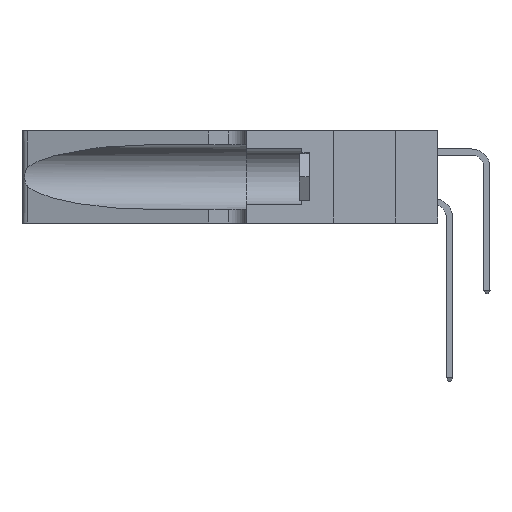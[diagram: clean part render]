
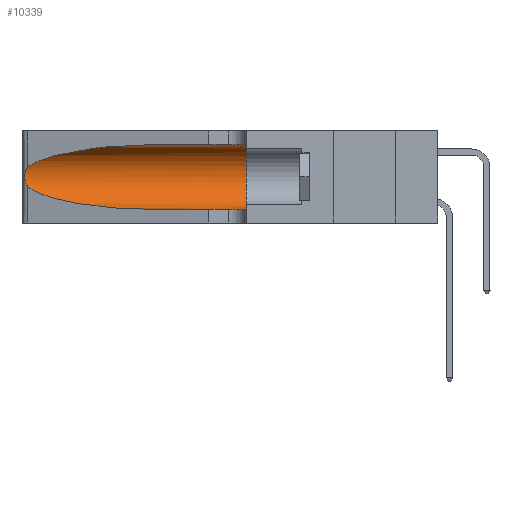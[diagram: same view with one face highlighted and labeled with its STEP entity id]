
A CAD part, left-side view. The second image highlights one B-rep face of the part: STEP entity #10339.
In plain terms, the highlighted cylindrical face has radius 3.308 mm (diameter 6.617 mm), a partial arc.
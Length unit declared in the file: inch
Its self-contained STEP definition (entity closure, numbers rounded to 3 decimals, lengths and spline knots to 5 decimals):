
#837 =( BOUNDED_CURVE ( )  B_SPLINE_CURVE ( 3, ( #22270, #9101, #14815, #3333 ),
 .UNSPECIFIED., .F., .T. ) 
 B_SPLINE_CURVE_WITH_KNOTS ( ( 4, 4 ),
 ( 1.5708, 2.84003 ),
 .UNSPECIFIED. ) 
 CURVE ( )  GEOMETRIC_REPRESENTATION_ITEM ( )  RATIONAL_B_SPLINE_CURVE ( ( 1., 0.87, 0.87, 1. ) ) 
 REPRESENTATION_ITEM ( '' )  );
#998 = EDGE_CURVE ( 'NONE', #23473, #14423, #1477, .T. ) ;
#1050 = ORIENTED_EDGE ( 'NONE', *, *, #11683, .T. ) ;
#1198 = EDGE_CURVE ( 'NONE', #12039, #12896, #8550, .T. ) ;
#1477 = B_SPLINE_CURVE_WITH_KNOTS ( 'NONE', 3,
 ( #12448, #19894, #19383, #19807, #13295, #18760, #21488, #17573, #22942, #7159, #22760, #13082, #13023, #12471 ),
 .UNSPECIFIED., .F., .F.,
 ( 4, 2, 2, 2, 2, 2, 4 ),
 ( 0., 0.00027, 0.00053, 0.00107, 0.0016, 0.00187, 0.00214 ),
 .UNSPECIFIED. ) ;
#3090 = EDGE_CURVE ( 'NONE', #20179, #12896, #11149, .T. ) ;
#3333 = CARTESIAN_POINT ( 'NONE',  ( 0.25487, 1.22718, 0.22369 ) ) ;
#4627 = CARTESIAN_POINT ( 'NONE',  ( 0.1305, 0.72297, 0.05475 ) ) ;
#5483 = CARTESIAN_POINT ( 'NONE',  ( 0.25487, 1.22718, 0.14631 ) ) ;
#5900 = ORIENTED_EDGE ( 'NONE', *, *, #1198, .T. ) ;
#6543 = CARTESIAN_POINT ( 'NONE',  ( 0.1305, 1.61858, 0.185 ) ) ;
#7159 = CARTESIAN_POINT ( 'NONE',  ( 0.25856, 1.23593, 0.16098 ) ) ;
#7175 = ORIENTED_EDGE ( 'NONE', *, *, #23449, .F. ) ;
#7817 = CARTESIAN_POINT ( 'NONE',  ( 0.1305, 1.61858, 0.05475 ) ) ;
#8189 = AXIS2_PLACEMENT_3D ( 'NONE', #20800, #9505, #22675 ) ;
#8471 = DIRECTION ( 'NONE',  ( 0., -1., 0. ) ) ;
#8550 = LINE ( 'NONE', #7817, #22967 ) ;
#9101 = CARTESIAN_POINT ( 'NONE',  ( 0.18966, 0.96281, 0.31525 ) ) ;
#9147 = EDGE_LOOP ( 'NONE', ( #11812, #12582, #1050, #5900, #21567, #7175 ) ) ;
#9505 = DIRECTION ( 'NONE',  ( 0., 1., 0. ) ) ;
#10339 = ADVANCED_FACE ( 'NONE', ( #23622 ), #13663, .F. ) ;
#10378 = CARTESIAN_POINT ( 'NONE',  ( 0.25487, 1.22718, 0.14631 ) ) ;
#11149 = CIRCLE ( 'NONE', #8189, 0.13025 ) ;
#11683 = EDGE_CURVE ( 'NONE', #14423, #12039, #18564, .T. ) ;
#11812 = ORIENTED_EDGE ( 'NONE', *, *, #18090, .T. ) ;
#12039 = VERTEX_POINT ( 'NONE', #21020 ) ;
#12448 = CARTESIAN_POINT ( 'NONE',  ( 0.25487, 1.22718, 0.22369 ) ) ;
#12471 = CARTESIAN_POINT ( 'NONE',  ( 0.25487, 1.22718, 0.14631 ) ) ;
#12582 = ORIENTED_EDGE ( 'NONE', *, *, #998, .T. ) ;
#12896 = VERTEX_POINT ( 'NONE', #18208 ) ;
#13023 = CARTESIAN_POINT ( 'NONE',  ( 0.25555, 1.22993, 0.14849 ) ) ;
#13082 = CARTESIAN_POINT ( 'NONE',  ( 0.25639, 1.23186, 0.15144 ) ) ;
#13295 = CARTESIAN_POINT ( 'NONE',  ( 0.25854, 1.2359, 0.20912 ) ) ;
#13557 = CARTESIAN_POINT ( 'NONE',  ( 0.1305, 0.35, 0.31525 ) ) ;
#13663 = CYLINDRICAL_SURFACE ( 'NONE', #22860, 0.13025 ) ;
#14158 = DIRECTION ( 'NONE',  ( 0., 0., -1. ) ) ;
#14423 = VERTEX_POINT ( 'NONE', #5483 ) ;
#14815 = CARTESIAN_POINT ( 'NONE',  ( 0.2373, 1.15595, 0.28018 ) ) ;
#15953 = VERTEX_POINT ( 'NONE', #20890 ) ;
#16080 = CARTESIAN_POINT ( 'NONE',  ( 0.18966, 0.96281, 0.05475 ) ) ;
#17573 = CARTESIAN_POINT ( 'NONE',  ( 0.26075, 1.23896, 0.178 ) ) ;
#17799 = VECTOR ( 'NONE', #8471, 39.37008 ) ;
#17928 = DIRECTION ( 'NONE',  ( 0., -1., 0. ) ) ;
#18090 = EDGE_CURVE ( 'NONE', #15953, #23473, #837, .T. ) ;
#18198 = DIRECTION ( 'NONE',  ( 0., -1., 0. ) ) ;
#18208 = CARTESIAN_POINT ( 'NONE',  ( 0.1305, 0.35, 0.05475 ) ) ;
#18384 = LINE ( 'NONE', #23520, #17799 ) ;
#18564 =( BOUNDED_CURVE ( )  B_SPLINE_CURVE ( 3, ( #10378, #21641, #16080, #4627 ),
 .UNSPECIFIED., .F., .T. ) 
 B_SPLINE_CURVE_WITH_KNOTS ( ( 4, 4 ),
 ( 3.44316, 4.71239 ),
 .UNSPECIFIED. ) 
 CURVE ( )  GEOMETRIC_REPRESENTATION_ITEM ( )  RATIONAL_B_SPLINE_CURVE ( ( 1., 0.87, 0.87, 1. ) ) 
 REPRESENTATION_ITEM ( '' )  );
#18760 = CARTESIAN_POINT ( 'NONE',  ( 0.26018, 1.23835, 0.19895 ) ) ;
#19383 = CARTESIAN_POINT ( 'NONE',  ( 0.25639, 1.23184, 0.21858 ) ) ;
#19807 = CARTESIAN_POINT ( 'NONE',  ( 0.25787, 1.23484, 0.2124 ) ) ;
#19894 = CARTESIAN_POINT ( 'NONE',  ( 0.25555, 1.22994, 0.2215 ) ) ;
#20179 = VERTEX_POINT ( 'NONE', #13557 ) ;
#20800 = CARTESIAN_POINT ( 'NONE',  ( 0.1305, 0.35, 0.185 ) ) ;
#20890 = CARTESIAN_POINT ( 'NONE',  ( 0.1305, 0.72297, 0.31525 ) ) ;
#21020 = CARTESIAN_POINT ( 'NONE',  ( 0.1305, 0.72297, 0.05475 ) ) ;
#21488 = CARTESIAN_POINT ( 'NONE',  ( 0.26075, 1.23896, 0.19203 ) ) ;
#21567 = ORIENTED_EDGE ( 'NONE', *, *, #3090, .F. ) ;
#21641 = CARTESIAN_POINT ( 'NONE',  ( 0.2373, 1.15595, 0.08982 ) ) ;
#21747 = CARTESIAN_POINT ( 'NONE',  ( 0.25487, 1.22718, 0.22369 ) ) ;
#22270 = CARTESIAN_POINT ( 'NONE',  ( 0.1305, 0.72297, 0.31525 ) ) ;
#22675 = DIRECTION ( 'NONE',  ( 0., 0., 1. ) ) ;
#22760 = CARTESIAN_POINT ( 'NONE',  ( 0.25789, 1.23486, 0.15765 ) ) ;
#22860 = AXIS2_PLACEMENT_3D ( 'NONE', #6543, #17928, #14158 ) ;
#22942 = CARTESIAN_POINT ( 'NONE',  ( 0.26017, 1.23833, 0.17102 ) ) ;
#22967 = VECTOR ( 'NONE', #18198, 39.37008 ) ;
#23449 = EDGE_CURVE ( 'NONE', #15953, #20179, #18384, .T. ) ;
#23473 = VERTEX_POINT ( 'NONE', #21747 ) ;
#23520 = CARTESIAN_POINT ( 'NONE',  ( 0.1305, 1.61858, 0.31525 ) ) ;
#23622 = FACE_OUTER_BOUND ( 'NONE', #9147, .T. ) ;
